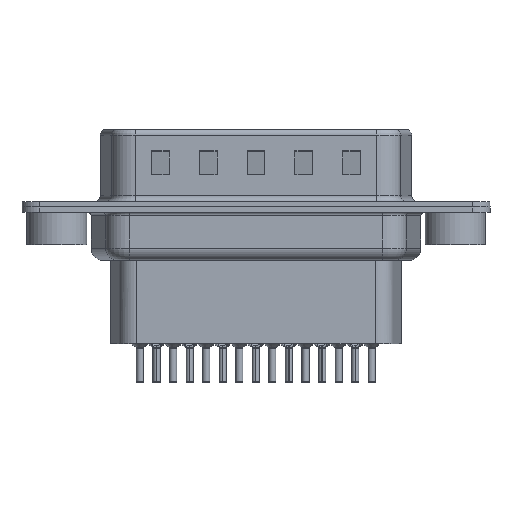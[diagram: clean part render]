
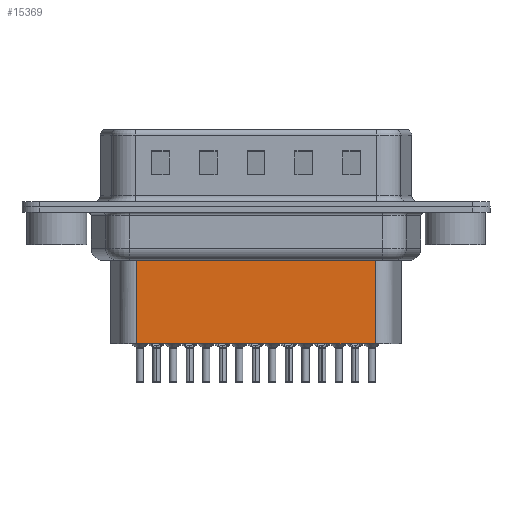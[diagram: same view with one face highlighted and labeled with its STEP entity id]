
A CAD part, front view. The second image highlights one B-rep face of the part: STEP entity #15369.
In plain terms, the highlighted planar face has unit normal (0, -1, 0).
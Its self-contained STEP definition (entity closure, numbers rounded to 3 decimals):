
#1788 = VERTEX_POINT ( 'NONE', #9767 ) ;
#1863 = VERTEX_POINT ( 'NONE', #15707 ) ;
#1931 = CARTESIAN_POINT ( 'NONE',  ( 6.434, -3.5, -4.097 ) ) ;
#2083 = VERTEX_POINT ( 'NONE', #14880 ) ;
#2225 = ORIENTED_EDGE ( 'NONE', *, *, #5192, .T. ) ;
#2318 = CARTESIAN_POINT ( 'NONE',  ( 26.619, -3.5, -3.1 ) ) ;
#3006 = DIRECTION ( 'NONE',  ( -1., 0., 0. ) ) ;
#3545 = ORIENTED_EDGE ( 'NONE', *, *, #14369, .F. ) ;
#3762 = VECTOR ( 'NONE', #3006, 1000. ) ;
#4679 = ORIENTED_EDGE ( 'NONE', *, *, #12197, .F. ) ;
#5192 = EDGE_CURVE ( 'NONE', #1863, #1788, #12026, .T. ) ;
#5896 = VERTEX_POINT ( 'NONE', #7366 ) ;
#6688 = VECTOR ( 'NONE', #8864, 1000. ) ;
#6995 = VECTOR ( 'NONE', #18140, 1000. ) ;
#7204 = LINE ( 'NONE', #2318, #6688 ) ;
#7366 = CARTESIAN_POINT ( 'NONE',  ( 6.681, -3.5, -11.45 ) ) ;
#7663 = PLANE ( 'NONE',  #15731 ) ;
#7927 = LINE ( 'NONE', #21191, #10730 ) ;
#8393 = FACE_OUTER_BOUND ( 'NONE', #16964, .T. ) ;
#8864 = DIRECTION ( 'NONE',  ( 0., 0., -1. ) ) ;
#9767 = CARTESIAN_POINT ( 'NONE',  ( 6.681, -3.5, -4.097 ) ) ;
#9827 = DIRECTION ( 'NONE',  ( -1., 0., 0. ) ) ;
#10730 = VECTOR ( 'NONE', #9827, 1000. ) ;
#10949 = DIRECTION ( 'NONE',  ( 1., 0., 0. ) ) ;
#11366 = LINE ( 'NONE', #19713, #6995 ) ;
#12026 = LINE ( 'NONE', #1931, #3762 ) ;
#12197 = EDGE_CURVE ( 'NONE', #1863, #2083, #7204, .T. ) ;
#14369 = EDGE_CURVE ( 'NONE', #2083, #5896, #7927, .T. ) ;
#14880 = CARTESIAN_POINT ( 'NONE',  ( 26.619, -3.5, -11.45 ) ) ;
#15369 = ADVANCED_FACE ( 'NONE', ( #8393 ), #7663, .T. ) ;
#15707 = CARTESIAN_POINT ( 'NONE',  ( 26.619, -3.5, -4.097 ) ) ;
#15731 = AXIS2_PLACEMENT_3D ( 'NONE', #19009, #15786, #10949 ) ;
#15786 = DIRECTION ( 'NONE',  ( 0., -1., 0. ) ) ;
#16575 = ORIENTED_EDGE ( 'NONE', *, *, #18686, .T. ) ;
#16964 = EDGE_LOOP ( 'NONE', ( #4679, #2225, #16575, #3545 ) ) ;
#18140 = DIRECTION ( 'NONE',  ( 0., 0., -1. ) ) ;
#18686 = EDGE_CURVE ( 'NONE', #1788, #5896, #11366, .T. ) ;
#19009 = CARTESIAN_POINT ( 'NONE',  ( 6.681, -3.5, -3.1 ) ) ;
#19713 = CARTESIAN_POINT ( 'NONE',  ( 6.681, -3.5, -3.1 ) ) ;
#21191 = CARTESIAN_POINT ( 'NONE',  ( 6.681, -3.5, -11.45 ) ) ;
